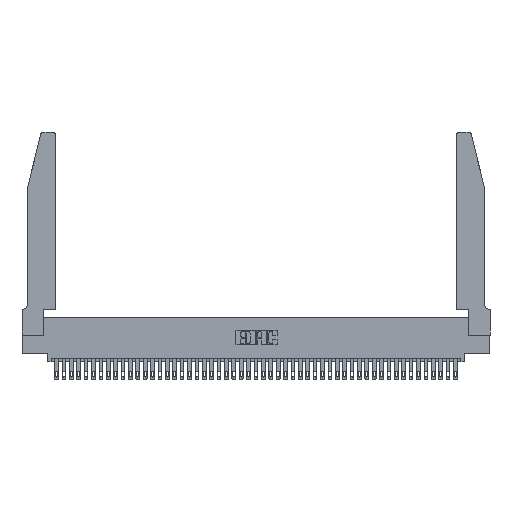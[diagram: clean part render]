
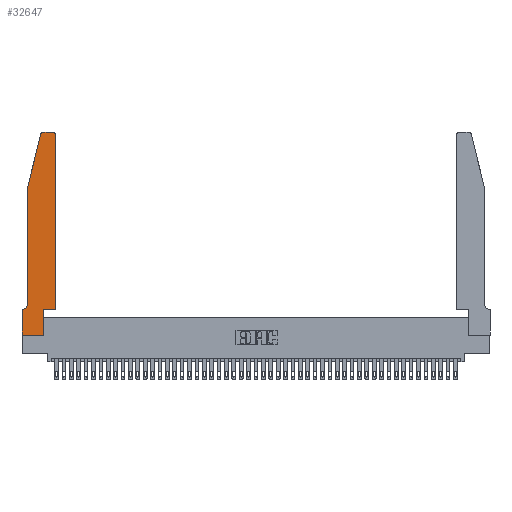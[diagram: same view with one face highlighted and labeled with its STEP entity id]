
A CAD part, top view. The second image highlights one B-rep face of the part: STEP entity #32647.
In plain terms, the highlighted planar face has unit normal (0, 0, 1).
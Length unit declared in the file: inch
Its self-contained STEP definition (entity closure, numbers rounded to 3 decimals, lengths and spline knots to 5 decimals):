
#236 = DIRECTION ( 'NONE',  ( 0., -1., 0. ) ) ;
#789 = CARTESIAN_POINT ( 'NONE',  ( 0.2865, 0.35, 0.37 ) ) ;
#847 = EDGE_CURVE ( 'NONE', #41129, #5766, #1484, .T. ) ;
#1254 = CARTESIAN_POINT ( 'NONE',  ( 0.0755, 2., 0.37 ) ) ;
#1484 = CIRCLE ( 'NONE', #35255, 0.03 ) ;
#1906 = VECTOR ( 'NONE', #20786, 39.37008 ) ;
#2856 = LINE ( 'NONE', #38304, #35831 ) ;
#2996 = DIRECTION ( 'NONE',  ( -1., 0., 0. ) ) ;
#4305 = VECTOR ( 'NONE', #8028, 39.37008 ) ;
#4804 = DIRECTION ( 'NONE',  ( -1., 0., 0. ) ) ;
#5766 = VERTEX_POINT ( 'NONE', #32380 ) ;
#6301 = LINE ( 'NONE', #32411, #12456 ) ;
#7564 = LINE ( 'NONE', #7599, #42206 ) ;
#7599 = CARTESIAN_POINT ( 'NONE',  ( 0., 0., 0.37 ) ) ;
#8028 = DIRECTION ( 'NONE',  ( 0., -1., 0. ) ) ;
#8050 = ORIENTED_EDGE ( 'NONE', *, *, #20983, .T. ) ;
#8525 = ORIENTED_EDGE ( 'NONE', *, *, #23112, .T. ) ;
#8760 = LINE ( 'NONE', #1254, #13243 ) ;
#9056 = CARTESIAN_POINT ( 'NONE',  ( 0.4205, 2.75, 0.37 ) ) ;
#10449 = AXIS2_PLACEMENT_3D ( 'NONE', #21802, #21650, #18035 ) ;
#10961 = EDGE_CURVE ( 'NONE', #40514, #41129, #42100, .T. ) ;
#11276 = DIRECTION ( 'NONE',  ( 1., 0., 0. ) ) ;
#11383 = LINE ( 'NONE', #13741, #1906 ) ;
#11501 = DIRECTION ( 'NONE',  ( 0., 0., -1. ) ) ;
#12142 = CARTESIAN_POINT ( 'NONE',  ( 0., 0.35, 0.37 ) ) ;
#12299 = CARTESIAN_POINT ( 'NONE',  ( 0.4505, 0.35, 0.37 ) ) ;
#12343 = LINE ( 'NONE', #45744, #29711 ) ;
#12456 = VECTOR ( 'NONE', #11276, 39.37008 ) ;
#12641 = EDGE_CURVE ( 'NONE', #24494, #38692, #6301, .T. ) ;
#13138 = ORIENTED_EDGE ( 'NONE', *, *, #45969, .T. ) ;
#13243 = VECTOR ( 'NONE', #14375, 39.37008 ) ;
#13603 = VECTOR ( 'NONE', #4804, 39.37008 ) ;
#13674 = ORIENTED_EDGE ( 'NONE', *, *, #22510, .T. ) ;
#13741 = CARTESIAN_POINT ( 'NONE',  ( 0.2865, 0.35, 0.37 ) ) ;
#13964 = CARTESIAN_POINT ( 'NONE',  ( 0.0755, 2., 0.37 ) ) ;
#14375 = DIRECTION ( 'NONE',  ( -0.239, -0.971, 0. ) ) ;
#14478 = DIRECTION ( 'NONE',  ( -1., 0., 0. ) ) ;
#14915 = VECTOR ( 'NONE', #40700, 39.37008 ) ;
#15005 = ORIENTED_EDGE ( 'NONE', *, *, #42044, .T. ) ;
#15394 = CARTESIAN_POINT ( 'NONE',  ( 0.0055, 0.35, 0.37 ) ) ;
#16069 = AXIS2_PLACEMENT_3D ( 'NONE', #35538, #46227, #28492 ) ;
#16281 = ORIENTED_EDGE ( 'NONE', *, *, #35920, .T. ) ;
#16522 = ORIENTED_EDGE ( 'NONE', *, *, #21009, .T. ) ;
#16769 = FACE_OUTER_BOUND ( 'NONE', #31183, .T. ) ;
#17048 = VERTEX_POINT ( 'NONE', #19759 ) ;
#18035 = DIRECTION ( 'NONE',  ( 1., 0., 0. ) ) ;
#18434 = CARTESIAN_POINT ( 'NONE',  ( 0.0755, 0.42, 0.37 ) ) ;
#19759 = CARTESIAN_POINT ( 'NONE',  ( 0.4505, 0.35, 0.37 ) ) ;
#20786 = DIRECTION ( 'NONE',  ( 0., 1., 0. ) ) ;
#20983 = EDGE_CURVE ( 'NONE', #38681, #43149, #34994, .T. ) ;
#21009 = EDGE_CURVE ( 'NONE', #45022, #24494, #7564, .T. ) ;
#21443 = CARTESIAN_POINT ( 'NONE',  ( 0.4505, 2.72, 0.37 ) ) ;
#21650 = DIRECTION ( 'NONE',  ( 0., 0., 1. ) ) ;
#21802 = CARTESIAN_POINT ( 'NONE',  ( 0.4205, 2.72, 0.37 ) ) ;
#22189 = LINE ( 'NONE', #12299, #14915 ) ;
#22510 = EDGE_CURVE ( 'NONE', #24416, #38681, #44058, .T. ) ;
#23112 = EDGE_CURVE ( 'NONE', #5766, #24416, #8760, .T. ) ;
#24416 = VERTEX_POINT ( 'NONE', #13964 ) ;
#24494 = VERTEX_POINT ( 'NONE', #43773 ) ;
#27143 = EDGE_CURVE ( 'NONE', #17048, #43388, #22189, .T. ) ;
#27266 = CARTESIAN_POINT ( 'NONE',  ( 0.284, 2.75, 0.37 ) ) ;
#27982 = ORIENTED_EDGE ( 'NONE', *, *, #10961, .T. ) ;
#28492 = DIRECTION ( 'NONE',  ( 1., 0., 0. ) ) ;
#28774 = ORIENTED_EDGE ( 'NONE', *, *, #847, .T. ) ;
#29711 = VECTOR ( 'NONE', #2996, 39.37008 ) ;
#30147 = CARTESIAN_POINT ( 'NONE',  ( 0.2605, 2.75, 0.37 ) ) ;
#31183 = EDGE_LOOP ( 'NONE', ( #27982, #28774, #8525, #13674, #8050, #13138, #16522, #44354, #15005, #44149, #42603, #16281 ) ) ;
#32109 = PLANE ( 'NONE',  #16069 ) ;
#32380 = CARTESIAN_POINT ( 'NONE',  ( 0.25487, 2.72718, 0.37 ) ) ;
#32411 = CARTESIAN_POINT ( 'NONE',  ( 0., 0., 0.37 ) ) ;
#32647 = ADVANCED_FACE ( 'NONE', ( #16769 ), #32109, .T. ) ;
#32789 = CARTESIAN_POINT ( 'NONE',  ( 0.0055, 0.42, 0.37 ) ) ;
#33881 = CARTESIAN_POINT ( 'NONE',  ( 0.284, 2.72, 0.37 ) ) ;
#34179 = DIRECTION ( 'NONE',  ( 0., 0., 1. ) ) ;
#34659 = AXIS2_PLACEMENT_3D ( 'NONE', #32789, #11501, #14478 ) ;
#34994 = CIRCLE ( 'NONE', #34659, 0.07 ) ;
#35046 = DIRECTION ( 'NONE',  ( 1., 0., 0. ) ) ;
#35255 = AXIS2_PLACEMENT_3D ( 'NONE', #33881, #34179, #44298 ) ;
#35538 = CARTESIAN_POINT ( 'NONE',  ( 0., 0.35, 0.37 ) ) ;
#35831 = VECTOR ( 'NONE', #35046, 39.37008 ) ;
#35920 = EDGE_CURVE ( 'NONE', #43388, #40514, #37819, .T. ) ;
#37819 = CIRCLE ( 'NONE', #10449, 0.03 ) ;
#38304 = CARTESIAN_POINT ( 'NONE',  ( 0.4505, 0.35, 0.37 ) ) ;
#38681 = VERTEX_POINT ( 'NONE', #18434 ) ;
#38692 = VERTEX_POINT ( 'NONE', #43277 ) ;
#39262 = CARTESIAN_POINT ( 'NONE',  ( 0.0755, 2., 0.37 ) ) ;
#40009 = VERTEX_POINT ( 'NONE', #789 ) ;
#40514 = VERTEX_POINT ( 'NONE', #9056 ) ;
#40700 = DIRECTION ( 'NONE',  ( 0., 1., 0. ) ) ;
#41129 = VERTEX_POINT ( 'NONE', #27266 ) ;
#42044 = EDGE_CURVE ( 'NONE', #38692, #40009, #11383, .T. ) ;
#42100 = LINE ( 'NONE', #30147, #13603 ) ;
#42206 = VECTOR ( 'NONE', #236, 39.37008 ) ;
#42603 = ORIENTED_EDGE ( 'NONE', *, *, #27143, .T. ) ;
#43149 = VERTEX_POINT ( 'NONE', #15394 ) ;
#43277 = CARTESIAN_POINT ( 'NONE',  ( 0.2865, 0., 0.37 ) ) ;
#43388 = VERTEX_POINT ( 'NONE', #21443 ) ;
#43773 = CARTESIAN_POINT ( 'NONE',  ( 0., 0., 0.37 ) ) ;
#44058 = LINE ( 'NONE', #39262, #4305 ) ;
#44149 = ORIENTED_EDGE ( 'NONE', *, *, #45840, .T. ) ;
#44298 = DIRECTION ( 'NONE',  ( 1., 0., 0. ) ) ;
#44354 = ORIENTED_EDGE ( 'NONE', *, *, #12641, .T. ) ;
#45022 = VERTEX_POINT ( 'NONE', #12142 ) ;
#45744 = CARTESIAN_POINT ( 'NONE',  ( 0.0755, 0.35, 0.37 ) ) ;
#45840 = EDGE_CURVE ( 'NONE', #40009, #17048, #2856, .T. ) ;
#45969 = EDGE_CURVE ( 'NONE', #43149, #45022, #12343, .T. ) ;
#46227 = DIRECTION ( 'NONE',  ( 0., 0., 1. ) ) ;
